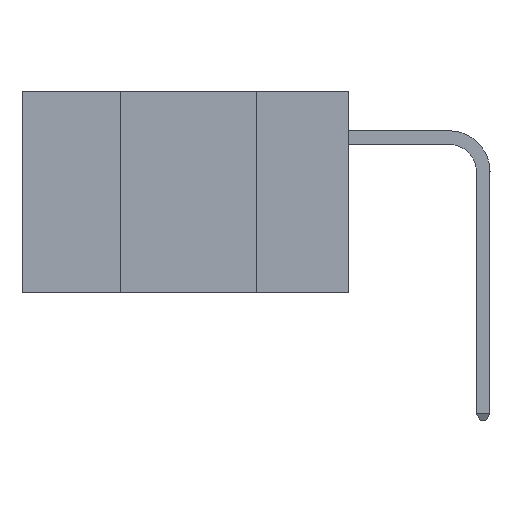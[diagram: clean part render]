
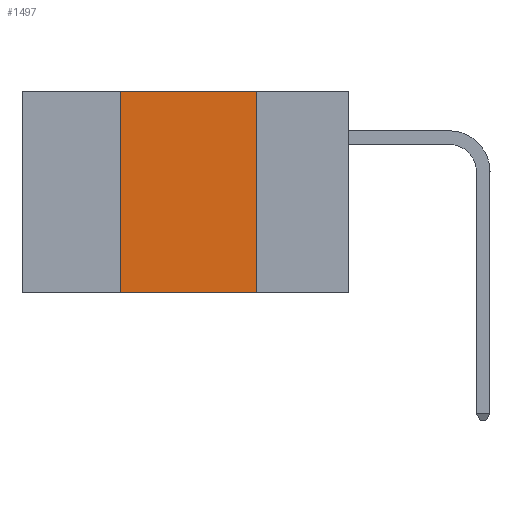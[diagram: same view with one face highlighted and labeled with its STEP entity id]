
A CAD part, left-side view. The second image highlights one B-rep face of the part: STEP entity #1497.
In plain terms, the highlighted planar face has unit normal (-1, 0, 0).
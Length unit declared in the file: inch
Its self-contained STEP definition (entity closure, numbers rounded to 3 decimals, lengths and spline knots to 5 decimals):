
#9 = VECTOR ( 'NONE', #9631, 39.37008 ) ;
#704 = CARTESIAN_POINT ( 'NONE',  ( 0., 0.42, -0.37 ) ) ;
#752 = FACE_OUTER_BOUND ( 'NONE', #3138, .T. ) ;
#1209 = LINE ( 'NONE', #12340, #7630 ) ;
#1497 = ADVANCED_FACE ( 'NONE', ( #752 ), #11998, .F. ) ;
#2337 = CARTESIAN_POINT ( 'NONE',  ( 0., 0.17, 0. ) ) ;
#3138 = EDGE_LOOP ( 'NONE', ( #4537, #9440, #6713, #11389 ) ) ;
#3172 = EDGE_CURVE ( 'NONE', #11645, #8181, #1209, .T. ) ;
#3403 = CARTESIAN_POINT ( 'NONE',  ( 0., 0.42, 0. ) ) ;
#4529 = DIRECTION ( 'NONE',  ( 0., -1., 0. ) ) ;
#4537 = ORIENTED_EDGE ( 'NONE', *, *, #7831, .F. ) ;
#5480 = CARTESIAN_POINT ( 'NONE',  ( 0., 0.17, 0. ) ) ;
#5860 = CARTESIAN_POINT ( 'NONE',  ( 0., 0.6, 0. ) ) ;
#5994 = DIRECTION ( 'NONE',  ( 1., 0., 0. ) ) ;
#6308 = DIRECTION ( 'NONE',  ( 0., -1., 0. ) ) ;
#6713 = ORIENTED_EDGE ( 'NONE', *, *, #11056, .F. ) ;
#7450 = VECTOR ( 'NONE', #4529, 39.37008 ) ;
#7567 = CARTESIAN_POINT ( 'NONE',  ( 0., 0.6, -0.37 ) ) ;
#7630 = VECTOR ( 'NONE', #6308, 39.37008 ) ;
#7831 = EDGE_CURVE ( 'NONE', #8181, #8598, #10505, .T. ) ;
#7921 = DIRECTION ( 'NONE',  ( 0., 0., -1. ) ) ;
#8181 = VERTEX_POINT ( 'NONE', #2337 ) ;
#8441 = LINE ( 'NONE', #3403, #9 ) ;
#8598 = VERTEX_POINT ( 'NONE', #10474 ) ;
#8692 = AXIS2_PLACEMENT_3D ( 'NONE', #5860, #5994, #7921 ) ;
#9440 = ORIENTED_EDGE ( 'NONE', *, *, #3172, .F. ) ;
#9513 = DIRECTION ( 'NONE',  ( 0., 0., -1. ) ) ;
#9532 = VERTEX_POINT ( 'NONE', #704 ) ;
#9631 = DIRECTION ( 'NONE',  ( 0., 0., 1. ) ) ;
#10474 = CARTESIAN_POINT ( 'NONE',  ( 0., 0.17, -0.37 ) ) ;
#10505 = LINE ( 'NONE', #5480, #10806 ) ;
#10543 = LINE ( 'NONE', #7567, #7450 ) ;
#10806 = VECTOR ( 'NONE', #9513, 39.37008 ) ;
#11056 = EDGE_CURVE ( 'NONE', #9532, #11645, #8441, .T. ) ;
#11389 = ORIENTED_EDGE ( 'NONE', *, *, #12893, .T. ) ;
#11645 = VERTEX_POINT ( 'NONE', #11926 ) ;
#11926 = CARTESIAN_POINT ( 'NONE',  ( 0., 0.42, 0. ) ) ;
#11998 = PLANE ( 'NONE',  #8692 ) ;
#12340 = CARTESIAN_POINT ( 'NONE',  ( 0., 0.6, 0. ) ) ;
#12893 = EDGE_CURVE ( 'NONE', #9532, #8598, #10543, .T. ) ;
